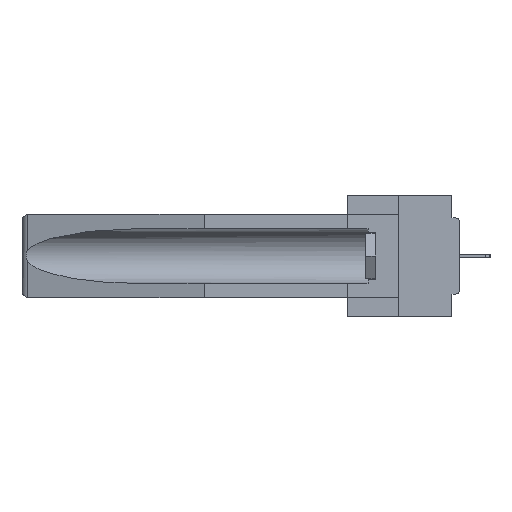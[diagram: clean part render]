
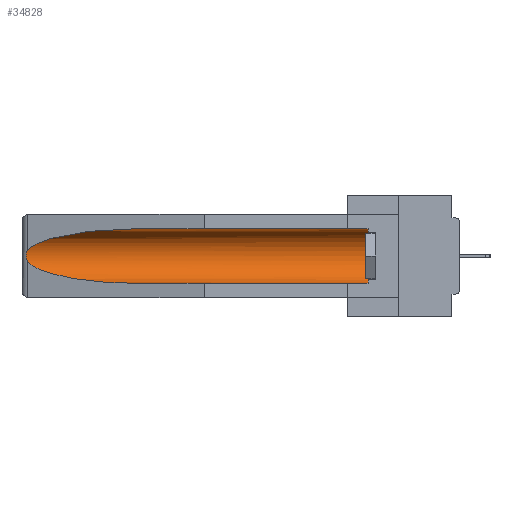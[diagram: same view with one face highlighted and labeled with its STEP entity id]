
A CAD part, left-side view. The second image highlights one B-rep face of the part: STEP entity #34828.
In plain terms, the highlighted cylindrical face has radius 2.857 mm (diameter 5.715 mm), a partial arc.
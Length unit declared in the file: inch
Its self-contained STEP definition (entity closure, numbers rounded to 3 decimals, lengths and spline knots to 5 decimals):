
#95 = CARTESIAN_POINT ( 'NONE',  ( 0.155, 0.126, -0.059 ) ) ;
#1707 = ORIENTED_EDGE ( 'NONE', *, *, #29012, .T. ) ;
#2959 = VERTEX_POINT ( 'NONE', #12636 ) ;
#3881 = ORIENTED_EDGE ( 'NONE', *, *, #4050, .T. ) ;
#4038 = ORIENTED_EDGE ( 'NONE', *, *, #11969, .T. ) ;
#4050 = EDGE_CURVE ( 'NONE', #2959, #16658, #11234, .T. ) ;
#4304 = CARTESIAN_POINT ( 'NONE',  ( 0.155, 0.126, -0.284 ) ) ;
#5078 = DIRECTION ( 'NONE',  ( 0., 1., 0. ) ) ;
#5996 = EDGE_CURVE ( 'NONE', #12689, #12466, #28883, .T. ) ;
#6638 = AXIS2_PLACEMENT_3D ( 'NONE', #21171, #24153, #18375 ) ;
#6927 = CARTESIAN_POINT ( 'NONE',  ( 0.155, 1.07973, -0.284 ) ) ;
#7824 = CARTESIAN_POINT ( 'NONE',  ( 0.26537, 1.52718, -0.14972 ) ) ;
#8582 = CARTESIAN_POINT ( 'NONE',  ( 0.155, 1.07973, -0.059 ) ) ;
#8670 = ORIENTED_EDGE ( 'NONE', *, *, #5996, .T. ) ;
#9440 = ORIENTED_EDGE ( 'NONE', *, *, #27309, .F. ) ;
#10778 = CARTESIAN_POINT ( 'NONE',  ( 0.2673, 1.53269, -0.17917 ) ) ;
#11147 = CARTESIAN_POINT ( 'NONE',  ( 0.26655, 1.53094, -0.18657 ) ) ;
#11234 =( BOUNDED_CURVE ( )  B_SPLINE_CURVE ( 3, ( #8582, #28505, #28695, #20293 ),
 .UNSPECIFIED., .F., .F. ) 
 B_SPLINE_CURVE_WITH_KNOTS ( ( 4, 4 ),
 ( 4.71239, 6.08839 ),
 .UNSPECIFIED. ) 
 CURVE ( )  GEOMETRIC_REPRESENTATION_ITEM ( )  RATIONAL_B_SPLINE_CURVE ( ( 1., 0.848, 0.848, 1. ) ) 
 REPRESENTATION_ITEM ( '' )  );
#11251 = CIRCLE ( 'NONE', #23159, 0.1125 ) ;
#11969 = EDGE_CURVE ( 'NONE', #13697, #2959, #33162, .T. ) ;
#12466 = VERTEX_POINT ( 'NONE', #24367 ) ;
#12636 = CARTESIAN_POINT ( 'NONE',  ( 0.155, 1.07973, -0.059 ) ) ;
#12689 = VERTEX_POINT ( 'NONE', #29217 ) ;
#13697 = VERTEX_POINT ( 'NONE', #95 ) ;
#13922 = CARTESIAN_POINT ( 'NONE',  ( 0.26597, 1.5296, -0.19026 ) ) ;
#15267 = CARTESIAN_POINT ( 'NONE',  ( 0.26537, 1.52718, -0.19328 ) ) ;
#15581 = FACE_OUTER_BOUND ( 'NONE', #26153, .T. ) ;
#16658 = VERTEX_POINT ( 'NONE', #16841 ) ;
#16742 = CARTESIAN_POINT ( 'NONE',  ( 0.2673, 1.5327, -0.16383 ) ) ;
#16841 = CARTESIAN_POINT ( 'NONE',  ( 0.26537, 1.52718, -0.14972 ) ) ;
#18375 = DIRECTION ( 'NONE',  ( 0., 0., 1. ) ) ;
#18993 = CARTESIAN_POINT ( 'NONE',  ( 0.155, -0.30754, -0.059 ) ) ;
#19153 = CARTESIAN_POINT ( 'NONE',  ( 0.26597, 1.52961, -0.15275 ) ) ;
#20202 = VECTOR ( 'NONE', #5078, 39.37008 ) ;
#20293 = CARTESIAN_POINT ( 'NONE',  ( 0.26537, 1.52718, -0.14972 ) ) ;
#20668 = CARTESIAN_POINT ( 'NONE',  ( 0.155, 0.126, -0.1715 ) ) ;
#21171 = CARTESIAN_POINT ( 'NONE',  ( 0.155, -0.30754, -0.1715 ) ) ;
#22443 = VECTOR ( 'NONE', #34914, 39.37008 ) ;
#23159 = AXIS2_PLACEMENT_3D ( 'NONE', #20668, #28566, #28377 ) ;
#24153 = DIRECTION ( 'NONE',  ( 0., 1., 0. ) ) ;
#24367 = CARTESIAN_POINT ( 'NONE',  ( 0.155, 1.07973, -0.284 ) ) ;
#25304 = CARTESIAN_POINT ( 'NONE',  ( 0.26537, 1.52718, -0.19328 ) ) ;
#26153 = EDGE_LOOP ( 'NONE', ( #3881, #35675, #8670, #9440, #1707, #4038 ) ) ;
#26643 = CARTESIAN_POINT ( 'NONE',  ( 0.25451, 1.48313, -0.24835 ) ) ;
#27309 = EDGE_CURVE ( 'NONE', #29242, #12466, #31944, .T. ) ;
#28377 = DIRECTION ( 'NONE',  ( 0., 0., 1. ) ) ;
#28505 = CARTESIAN_POINT ( 'NONE',  ( 0.21114, 1.30732, -0.059 ) ) ;
#28566 = DIRECTION ( 'NONE',  ( 0., -1., 0. ) ) ;
#28695 = CARTESIAN_POINT ( 'NONE',  ( 0.25451, 1.48313, -0.09465 ) ) ;
#28883 =( BOUNDED_CURVE ( )  B_SPLINE_CURVE ( 3, ( #15267, #26643, #35196, #6927 ),
 .UNSPECIFIED., .F., .F. ) 
 B_SPLINE_CURVE_WITH_KNOTS ( ( 4, 4 ),
 ( 0.1948, 1.5708 ),
 .UNSPECIFIED. ) 
 CURVE ( )  GEOMETRIC_REPRESENTATION_ITEM ( )  RATIONAL_B_SPLINE_CURVE ( ( 1., 0.848, 0.848, 1. ) ) 
 REPRESENTATION_ITEM ( '' )  );
#29012 = EDGE_CURVE ( 'NONE', #29242, #13697, #11251, .T. ) ;
#29217 = CARTESIAN_POINT ( 'NONE',  ( 0.26537, 1.52718, -0.19328 ) ) ;
#29242 = VERTEX_POINT ( 'NONE', #4304 ) ;
#29582 = CYLINDRICAL_SURFACE ( 'NONE', #6638, 0.1125 ) ;
#30549 = CARTESIAN_POINT ( 'NONE',  ( 0.26654, 1.53092, -0.15636 ) ) ;
#31296 = B_SPLINE_CURVE_WITH_KNOTS ( 'NONE', 3,
 ( #7824, #19153, #30549, #16742, #36283, #33129, #10778, #11147, #13922, #25304 ),
 .UNSPECIFIED., .F., .F.,
 ( 4, 2, 2, 2, 4 ),
 ( 0., 0.00029, 0.00058, 0.00087, 0.00117 ),
 .UNSPECIFIED. ) ;
#31590 = CARTESIAN_POINT ( 'NONE',  ( 0.155, -0.30754, -0.284 ) ) ;
#31944 = LINE ( 'NONE', #31590, #22443 ) ;
#32036 = EDGE_CURVE ( 'NONE', #16658, #12689, #31296, .T. ) ;
#33129 = CARTESIAN_POINT ( 'NONE',  ( 0.2675, 1.53308, -0.17534 ) ) ;
#33162 = LINE ( 'NONE', #18993, #20202 ) ;
#34828 = ADVANCED_FACE ( 'NONE', ( #15581 ), #29582, .F. ) ;
#34914 = DIRECTION ( 'NONE',  ( 0., 1., 0. ) ) ;
#35196 = CARTESIAN_POINT ( 'NONE',  ( 0.21114, 1.30732, -0.284 ) ) ;
#35675 = ORIENTED_EDGE ( 'NONE', *, *, #32036, .T. ) ;
#36283 = CARTESIAN_POINT ( 'NONE',  ( 0.2675, 1.53308, -0.16763 ) ) ;
